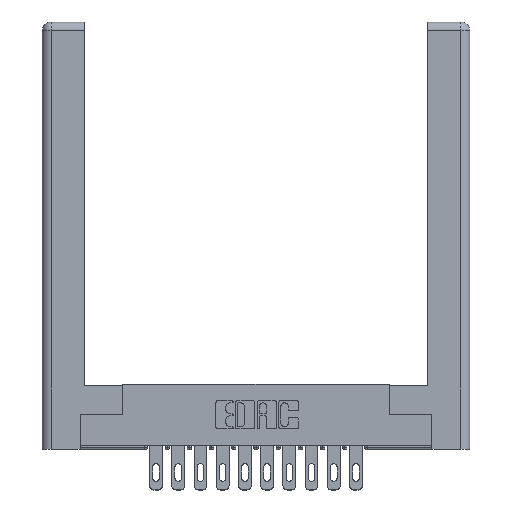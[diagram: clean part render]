
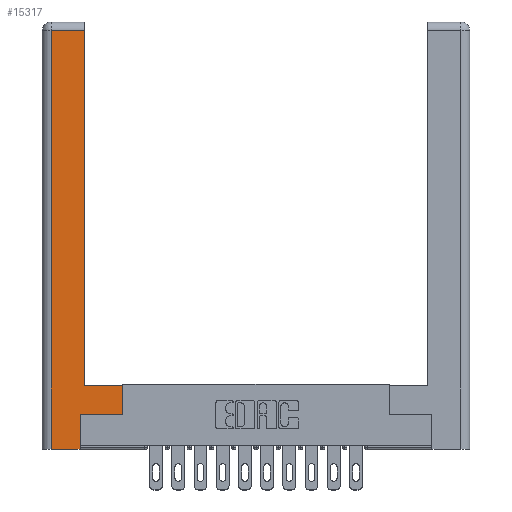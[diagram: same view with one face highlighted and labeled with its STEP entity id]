
A CAD part, top view. The second image highlights one B-rep face of the part: STEP entity #15317.
In plain terms, the highlighted planar face has unit normal (0, 0, 1).
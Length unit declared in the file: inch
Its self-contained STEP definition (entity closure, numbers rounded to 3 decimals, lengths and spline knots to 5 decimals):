
#9 = VECTOR ( 'NONE', #13961, 39.37008 ) ;
#38 = VERTEX_POINT ( 'NONE', #15263 ) ;
#271 = CARTESIAN_POINT ( 'NONE',  ( 0.0615, 0., 0. ) ) ;
#345 = VERTEX_POINT ( 'NONE', #2160 ) ;
#787 = EDGE_CURVE ( 'NONE', #7148, #6650, #13692, .T. ) ;
#1404 = EDGE_LOOP ( 'NONE', ( #15651, #11624, #15578, #6804, #10168, #12881, #5785, #3682 ) ) ;
#1568 = LINE ( 'NONE', #14331, #17100 ) ;
#1835 = LINE ( 'NONE', #271, #10702 ) ;
#2160 = CARTESIAN_POINT ( 'NONE',  ( 0.295, 2.94, 0. ) ) ;
#2302 = CARTESIAN_POINT ( 'NONE',  ( 0.565, 0.245, 0. ) ) ;
#2688 = VERTEX_POINT ( 'NONE', #13207 ) ;
#2919 = DIRECTION ( 'NONE',  ( 0., 1., 0. ) ) ;
#3097 = CARTESIAN_POINT ( 'NONE',  ( 0.295, 0.45, 0. ) ) ;
#3445 = AXIS2_PLACEMENT_3D ( 'NONE', #13655, #16747, #8857 ) ;
#3682 = ORIENTED_EDGE ( 'NONE', *, *, #787, .T. ) ;
#4238 = EDGE_CURVE ( 'NONE', #38, #8066, #1568, .T. ) ;
#4245 = PLANE ( 'NONE',  #3445 ) ;
#4367 = VECTOR ( 'NONE', #17256, 39.37008 ) ;
#5271 = DIRECTION ( 'NONE',  ( 1., 0., 0. ) ) ;
#5740 = FACE_OUTER_BOUND ( 'NONE', #1404, .T. ) ;
#5785 = ORIENTED_EDGE ( 'NONE', *, *, #9618, .T. ) ;
#6108 = LINE ( 'NONE', #10560, #12859 ) ;
#6123 = LINE ( 'NONE', #11404, #9 ) ;
#6218 = VERTEX_POINT ( 'NONE', #2302 ) ;
#6650 = VERTEX_POINT ( 'NONE', #11280 ) ;
#6737 = LINE ( 'NONE', #9614, #13474 ) ;
#6804 = ORIENTED_EDGE ( 'NONE', *, *, #4238, .T. ) ;
#7148 = VERTEX_POINT ( 'NONE', #8457 ) ;
#7355 = LINE ( 'NONE', #12524, #17176 ) ;
#7769 = CARTESIAN_POINT ( 'NONE',  ( 0.265, 0., 0. ) ) ;
#8021 = EDGE_CURVE ( 'NONE', #345, #2688, #6123, .T. ) ;
#8066 = VERTEX_POINT ( 'NONE', #7769 ) ;
#8457 = CARTESIAN_POINT ( 'NONE',  ( 0.565, 0.45, 0. ) ) ;
#8857 = DIRECTION ( 'NONE',  ( -1., 0., 0. ) ) ;
#9262 = LINE ( 'NONE', #15968, #4367 ) ;
#9613 = DIRECTION ( 'NONE',  ( 0., 1., 0. ) ) ;
#9614 = CARTESIAN_POINT ( 'NONE',  ( 0.265, 0.245, 0. ) ) ;
#9618 = EDGE_CURVE ( 'NONE', #6218, #7148, #6108, .T. ) ;
#9726 = EDGE_CURVE ( 'NONE', #6650, #345, #7355, .T. ) ;
#10168 = ORIENTED_EDGE ( 'NONE', *, *, #16616, .T. ) ;
#10361 = VECTOR ( 'NONE', #12607, 39.37008 ) ;
#10560 = CARTESIAN_POINT ( 'NONE',  ( 0.565, 0.45, 0. ) ) ;
#10615 = CARTESIAN_POINT ( 'NONE',  ( 0.265, 0.245, 0. ) ) ;
#10702 = VECTOR ( 'NONE', #15143, 39.37008 ) ;
#11280 = CARTESIAN_POINT ( 'NONE',  ( 0.295, 0.45, 0. ) ) ;
#11404 = CARTESIAN_POINT ( 'NONE',  ( 0.0615, 2.94, 0. ) ) ;
#11624 = ORIENTED_EDGE ( 'NONE', *, *, #8021, .T. ) ;
#12524 = CARTESIAN_POINT ( 'NONE',  ( 0.295, 3., 0. ) ) ;
#12607 = DIRECTION ( 'NONE',  ( -1., 0., 0. ) ) ;
#12859 = VECTOR ( 'NONE', #17067, 39.37008 ) ;
#12881 = ORIENTED_EDGE ( 'NONE', *, *, #17182, .T. ) ;
#13207 = CARTESIAN_POINT ( 'NONE',  ( 0.0615, 2.94, 0. ) ) ;
#13474 = VECTOR ( 'NONE', #2919, 39.37008 ) ;
#13655 = CARTESIAN_POINT ( 'NONE',  ( 0., 0., 0. ) ) ;
#13692 = LINE ( 'NONE', #3097, #10361 ) ;
#13961 = DIRECTION ( 'NONE',  ( -1., 0., 0. ) ) ;
#14331 = CARTESIAN_POINT ( 'NONE',  ( 0.265, 0., 0. ) ) ;
#14437 = VERTEX_POINT ( 'NONE', #10615 ) ;
#15143 = DIRECTION ( 'NONE',  ( 0., -1., 0. ) ) ;
#15263 = CARTESIAN_POINT ( 'NONE',  ( 0.0615, 0., 0. ) ) ;
#15317 = ADVANCED_FACE ( 'NONE', ( #5740 ), #4245, .F. ) ;
#15578 = ORIENTED_EDGE ( 'NONE', *, *, #17351, .T. ) ;
#15651 = ORIENTED_EDGE ( 'NONE', *, *, #9726, .T. ) ;
#15968 = CARTESIAN_POINT ( 'NONE',  ( 0.565, 0.245, 0. ) ) ;
#16616 = EDGE_CURVE ( 'NONE', #8066, #14437, #6737, .T. ) ;
#16747 = DIRECTION ( 'NONE',  ( 0., 0., -1. ) ) ;
#17067 = DIRECTION ( 'NONE',  ( 0., 1., 0. ) ) ;
#17100 = VECTOR ( 'NONE', #5271, 39.37008 ) ;
#17176 = VECTOR ( 'NONE', #9613, 39.37008 ) ;
#17182 = EDGE_CURVE ( 'NONE', #14437, #6218, #9262, .T. ) ;
#17256 = DIRECTION ( 'NONE',  ( 1., 0., 0. ) ) ;
#17351 = EDGE_CURVE ( 'NONE', #2688, #38, #1835, .T. ) ;
